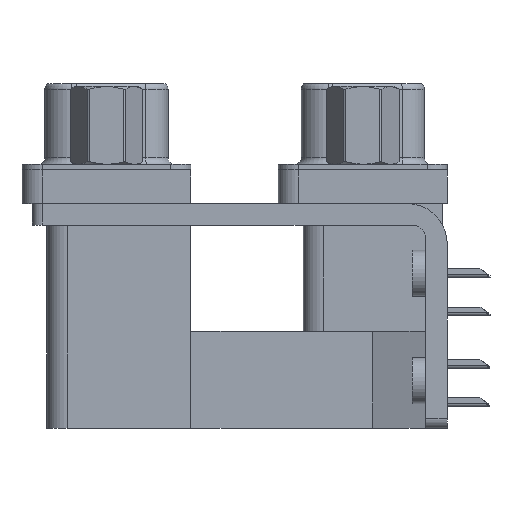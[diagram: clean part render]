
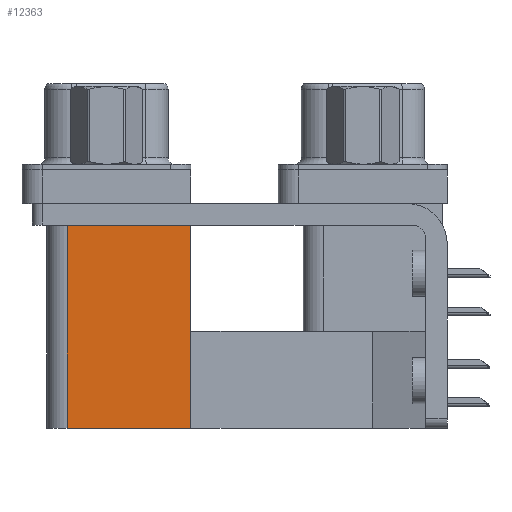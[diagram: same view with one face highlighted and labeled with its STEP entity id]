
A CAD part, left-side view. The second image highlights one B-rep face of the part: STEP entity #12363.
In plain terms, the highlighted planar face has unit normal (-1, 0, 0).
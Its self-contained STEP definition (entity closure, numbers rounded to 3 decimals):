
#1147 = DIRECTION ( 'NONE',  ( 0., 0., 1. ) ) ;
#2486 = PLANE ( 'NONE',  #7074 ) ;
#2875 = VERTEX_POINT ( 'NONE', #4223 ) ;
#4101 = EDGE_CURVE ( 'NONE', #2875, #10102, #22951, .T. ) ;
#4223 = CARTESIAN_POINT ( 'NONE',  ( 3.79, 21.975, -19.2 ) ) ;
#5006 = CARTESIAN_POINT ( 'NONE',  ( 3.79, 12.775, -19.2 ) ) ;
#5166 = DIRECTION ( 'NONE',  ( 1., 0., 0. ) ) ;
#7074 = AXIS2_PLACEMENT_3D ( 'NONE', #5006, #5166, #15203 ) ;
#8204 = CARTESIAN_POINT ( 'NONE',  ( 3.79, 12.775, -19.2 ) ) ;
#9414 = ORIENTED_EDGE ( 'NONE', *, *, #25426, .F. ) ;
#10102 = VERTEX_POINT ( 'NONE', #15778 ) ;
#10746 = VERTEX_POINT ( 'NONE', #8204 ) ;
#11716 = ORIENTED_EDGE ( 'NONE', *, *, #21758, .T. ) ;
#12363 = ADVANCED_FACE ( 'NONE', ( #16630 ), #2486, .F. ) ;
#12983 = VECTOR ( 'NONE', #23465, 1000. ) ;
#13429 = LINE ( 'NONE', #21447, #12983 ) ;
#13848 = DIRECTION ( 'NONE',  ( 0., 1., 0. ) ) ;
#13905 = CARTESIAN_POINT ( 'NONE',  ( 3.79, 12.775, -2.5 ) ) ;
#15203 = DIRECTION ( 'NONE',  ( 0., 0., -1. ) ) ;
#15778 = CARTESIAN_POINT ( 'NONE',  ( 3.79, 21.975, -2.5 ) ) ;
#16527 = CARTESIAN_POINT ( 'NONE',  ( 3.79, 12.775, -19.2 ) ) ;
#16630 = FACE_OUTER_BOUND ( 'NONE', #21910, .T. ) ;
#17044 = VECTOR ( 'NONE', #22792, 1000. ) ;
#17164 = ORIENTED_EDGE ( 'NONE', *, *, #4101, .F. ) ;
#17456 = EDGE_CURVE ( 'NONE', #10746, #32000, #22062, .T. ) ;
#18262 = CARTESIAN_POINT ( 'NONE',  ( 3.79, 21.975, -19.2 ) ) ;
#18844 = VECTOR ( 'NONE', #1147, 1000. ) ;
#18876 = CARTESIAN_POINT ( 'NONE',  ( 3.79, 12.775, -2.5 ) ) ;
#21380 = LINE ( 'NONE', #18876, #24015 ) ;
#21447 = CARTESIAN_POINT ( 'NONE',  ( 3.79, 12.775, -19.2 ) ) ;
#21758 = EDGE_CURVE ( 'NONE', #32000, #10102, #21380, .T. ) ;
#21910 = EDGE_LOOP ( 'NONE', ( #11716, #17164, #9414, #24204 ) ) ;
#22062 = LINE ( 'NONE', #16527, #18844 ) ;
#22792 = DIRECTION ( 'NONE',  ( 0., 0., 1. ) ) ;
#22951 = LINE ( 'NONE', #18262, #17044 ) ;
#23465 = DIRECTION ( 'NONE',  ( 0., 1., 0. ) ) ;
#24015 = VECTOR ( 'NONE', #13848, 1000. ) ;
#24204 = ORIENTED_EDGE ( 'NONE', *, *, #17456, .T. ) ;
#25426 = EDGE_CURVE ( 'NONE', #10746, #2875, #13429, .T. ) ;
#32000 = VERTEX_POINT ( 'NONE', #13905 ) ;
